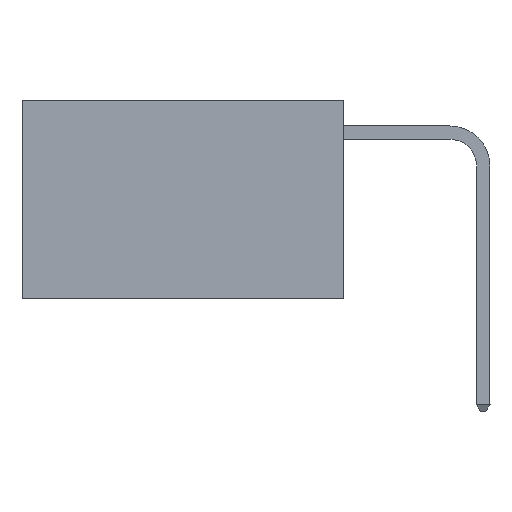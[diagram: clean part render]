
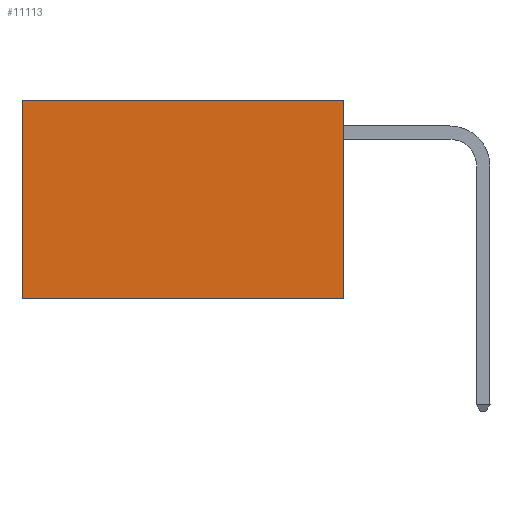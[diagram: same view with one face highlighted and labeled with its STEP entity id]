
A CAD part, left-side view. The second image highlights one B-rep face of the part: STEP entity #11113.
In plain terms, the highlighted planar face has unit normal (-1, 0, 0).
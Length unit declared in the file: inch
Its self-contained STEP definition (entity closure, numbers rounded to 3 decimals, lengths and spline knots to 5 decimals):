
#1904 = FACE_OUTER_BOUND ( 'NONE', #7261, .T. ) ;
#2217 = DIRECTION ( 'NONE',  ( 1., 0., 0. ) ) ;
#4194 = DIRECTION ( 'NONE',  ( 0., 0., -1. ) ) ;
#4552 = ORIENTED_EDGE ( 'NONE', *, *, #11880, .F. ) ;
#4938 = VECTOR ( 'NONE', #4194, 39.37008 ) ;
#5034 = ORIENTED_EDGE ( 'NONE', *, *, #16342, .T. ) ;
#5105 = PLANE ( 'NONE',  #15265 ) ;
#5206 = CARTESIAN_POINT ( 'NONE',  ( 0.2625, 0., 0. ) ) ;
#6556 = VECTOR ( 'NONE', #14459, 39.37008 ) ;
#7261 = EDGE_LOOP ( 'NONE', ( #14022, #15017, #4552, #5034 ) ) ;
#8789 = CARTESIAN_POINT ( 'NONE',  ( 0.2625, 0., -0.37 ) ) ;
#9277 = CARTESIAN_POINT ( 'NONE',  ( 0.2625, 0., 0. ) ) ;
#9781 = LINE ( 'NONE', #5206, #18045 ) ;
#10048 = VERTEX_POINT ( 'NONE', #16551 ) ;
#10498 = DIRECTION ( 'NONE',  ( 0., 1., 0. ) ) ;
#11113 = ADVANCED_FACE ( 'NONE', ( #1904 ), #5105, .F. ) ;
#11615 = EDGE_CURVE ( 'NONE', #13043, #20663, #13784, .T. ) ;
#11686 = DIRECTION ( 'NONE',  ( 0., 0., -1. ) ) ;
#11880 = EDGE_CURVE ( 'NONE', #19975, #13043, #9781, .T. ) ;
#13043 = VERTEX_POINT ( 'NONE', #20655 ) ;
#13784 = LINE ( 'NONE', #8789, #19369 ) ;
#14022 = ORIENTED_EDGE ( 'NONE', *, *, #18948, .T. ) ;
#14459 = DIRECTION ( 'NONE',  ( 0., 1., 0. ) ) ;
#15017 = ORIENTED_EDGE ( 'NONE', *, *, #11615, .F. ) ;
#15093 = CARTESIAN_POINT ( 'NONE',  ( 0.2625, 0., 0. ) ) ;
#15265 = AXIS2_PLACEMENT_3D ( 'NONE', #15093, #2217, #18300 ) ;
#16342 = EDGE_CURVE ( 'NONE', #19975, #10048, #19169, .T. ) ;
#16551 = CARTESIAN_POINT ( 'NONE',  ( 0.2625, 0.6, 0. ) ) ;
#17964 = CARTESIAN_POINT ( 'NONE',  ( 0.2625, 0.6, -0.37 ) ) ;
#18045 = VECTOR ( 'NONE', #11686, 39.37008 ) ;
#18300 = DIRECTION ( 'NONE',  ( 0., 0., -1. ) ) ;
#18586 = CARTESIAN_POINT ( 'NONE',  ( 0.2625, 0., 0. ) ) ;
#18948 = EDGE_CURVE ( 'NONE', #10048, #20663, #20048, .T. ) ;
#19169 = LINE ( 'NONE', #9277, #6556 ) ;
#19369 = VECTOR ( 'NONE', #10498, 39.37008 ) ;
#19975 = VERTEX_POINT ( 'NONE', #18586 ) ;
#20048 = LINE ( 'NONE', #20258, #4938 ) ;
#20258 = CARTESIAN_POINT ( 'NONE',  ( 0.2625, 0.6, 0. ) ) ;
#20655 = CARTESIAN_POINT ( 'NONE',  ( 0.2625, 0., -0.37 ) ) ;
#20663 = VERTEX_POINT ( 'NONE', #17964 ) ;
